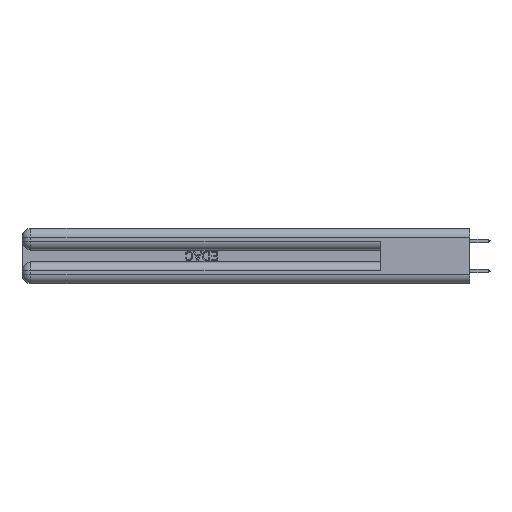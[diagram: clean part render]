
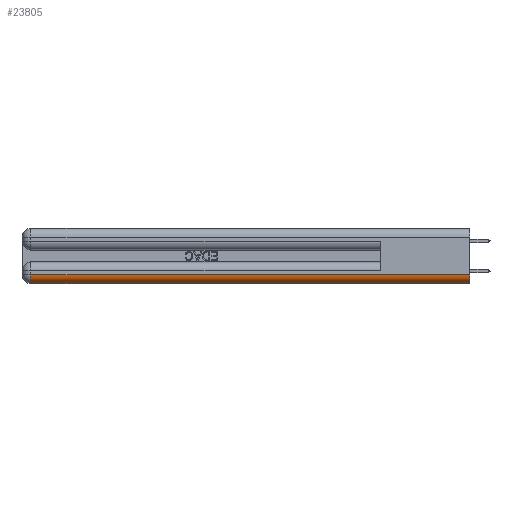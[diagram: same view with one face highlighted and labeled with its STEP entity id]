
A CAD part, left-side view. The second image highlights one B-rep face of the part: STEP entity #23805.
In plain terms, the highlighted cylindrical face has radius 1.524 mm (diameter 3.048 mm), a partial arc.
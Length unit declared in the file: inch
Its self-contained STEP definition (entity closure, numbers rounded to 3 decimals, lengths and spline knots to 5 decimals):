
#106 = VERTEX_POINT ( 'NONE', #45677 ) ;
#1877 = ORIENTED_EDGE ( 'NONE', *, *, #18908, .F. ) ;
#1931 = VECTOR ( 'NONE', #39213, 39.37008 ) ;
#3381 = EDGE_CURVE ( 'NONE', #21342, #14247, #28551, .T. ) ;
#4478 = LINE ( 'NONE', #23160, #1931 ) ;
#7459 = FACE_OUTER_BOUND ( 'NONE', #21640, .T. ) ;
#8968 = CARTESIAN_POINT ( 'NONE',  ( 0.06, 2.94, 0.06 ) ) ;
#9639 = CARTESIAN_POINT ( 'NONE',  ( 0., 0., 0.06 ) ) ;
#12996 = DIRECTION ( 'NONE',  ( 0., 0., 1. ) ) ;
#14247 = VERTEX_POINT ( 'NONE', #28846 ) ;
#17650 = CARTESIAN_POINT ( 'NONE',  ( 0., 0., 0.06 ) ) ;
#18353 = DIRECTION ( 'NONE',  ( 0., -1., 0. ) ) ;
#18908 = EDGE_CURVE ( 'NONE', #45588, #106, #47517, .T. ) ;
#21342 = VERTEX_POINT ( 'NONE', #17650 ) ;
#21640 = EDGE_LOOP ( 'NONE', ( #43713, #35769, #1877, #26618 ) ) ;
#22466 = AXIS2_PLACEMENT_3D ( 'NONE', #42266, #18353, #46280 ) ;
#23160 = CARTESIAN_POINT ( 'NONE',  ( 0.06, 3., 0. ) ) ;
#23805 = ADVANCED_FACE ( 'NONE', ( #7459 ), #27542, .T. ) ;
#26618 = ORIENTED_EDGE ( 'NONE', *, *, #32006, .F. ) ;
#27542 = CYLINDRICAL_SURFACE ( 'NONE', #41841, 0.06 ) ;
#28551 = CIRCLE ( 'NONE', #22466, 0.06 ) ;
#28846 = CARTESIAN_POINT ( 'NONE',  ( 0.06, 0., 0. ) ) ;
#30000 = CARTESIAN_POINT ( 'NONE',  ( 0.06, 2.94, 0. ) ) ;
#32006 = EDGE_CURVE ( 'NONE', #14247, #45588, #4478, .T. ) ;
#35398 = LINE ( 'NONE', #9639, #36662 ) ;
#35769 = ORIENTED_EDGE ( 'NONE', *, *, #37116, .F. ) ;
#36662 = VECTOR ( 'NONE', #37664, 39.37008 ) ;
#37018 = DIRECTION ( 'NONE',  ( 0., 1., 0. ) ) ;
#37116 = EDGE_CURVE ( 'NONE', #106, #21342, #35398, .T. ) ;
#37664 = DIRECTION ( 'NONE',  ( 0., -1., 0. ) ) ;
#39213 = DIRECTION ( 'NONE',  ( 0., 1., 0. ) ) ;
#39370 = DIRECTION ( 'NONE',  ( 0., 0., 1. ) ) ;
#41841 = AXIS2_PLACEMENT_3D ( 'NONE', #43366, #43187, #39370 ) ;
#42266 = CARTESIAN_POINT ( 'NONE',  ( 0.06, 0., 0.06 ) ) ;
#43187 = DIRECTION ( 'NONE',  ( 0., 1., 0. ) ) ;
#43366 = CARTESIAN_POINT ( 'NONE',  ( 0.06, 0., 0.06 ) ) ;
#43713 = ORIENTED_EDGE ( 'NONE', *, *, #3381, .F. ) ;
#45588 = VERTEX_POINT ( 'NONE', #30000 ) ;
#45677 = CARTESIAN_POINT ( 'NONE',  ( 0., 2.94, 0.06 ) ) ;
#46280 = DIRECTION ( 'NONE',  ( 0., 0., 1. ) ) ;
#47517 = CIRCLE ( 'NONE', #49732, 0.06 ) ;
#49732 = AXIS2_PLACEMENT_3D ( 'NONE', #8968, #37018, #12996 ) ;
